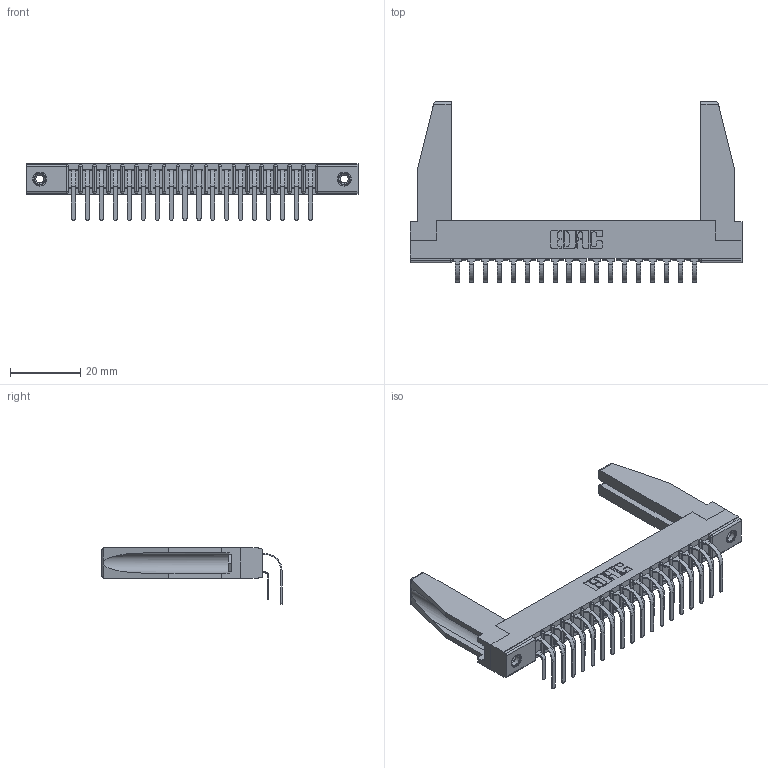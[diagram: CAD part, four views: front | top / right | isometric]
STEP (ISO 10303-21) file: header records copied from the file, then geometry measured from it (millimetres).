
FILE_DESCRIPTION (( 'STEP AP203' ), '1' );
FILE_NAME ('307-036-459-278.STEP', '2022-07-07T16:35:00', ( '' ), ( '' ), 'SwSTEP 2.0', 'SolidWorks 2020', '' );
FILE_SCHEMA (( 'CONFIG_CONTROL_DESIGN' ));
Length unit declared in the file: inch
Products named in the file (6): 307-290-001_558 559 - 1 (Single); 345-250-001_345-250-001-102; 307 Part_.156 Dia Mounting Holes; 307-036-459-278; 307-220-078; 307-290-001_559 - 2 (Single)
Assembly tree (41 placements, depth 2):
  307-036-459-278
    307 Part_.156 Dia Mounting Holes
    307-290-001_558 559 - 1 (Single)  x18
    307-290-001_559 - 2 (Single)  x18
    307-220-078  x2
    345-250-001_345-250-001-102  x2
Bounding box: 94.34 x 51.22 x 16.08 mm (x, y, z)
Volume: 10299.7 mm3; surface area: 15507.3 mm2
Topology: 41 solids, 41 shells, 2067 faces, 5765 edges, 3734 vertices
Faces by surface type: plane 1342, cylinder 671, sphere 38, cone 12, torus 4
Entity records: 22852 total; most frequent: CARTESIAN_POINT 3758, ORIENTED_EDGE 3680, DIRECTION 3644, EDGE_CURVE 1840, VECTOR 1404, LINE 1404, VERTEX_POINT 1192, AXIS2_PLACEMENT_3D 1120
